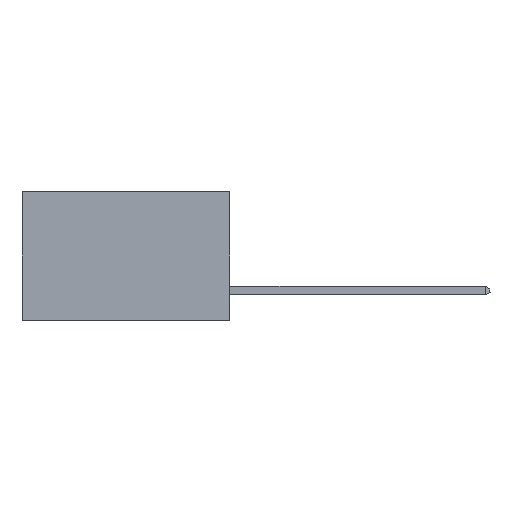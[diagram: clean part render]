
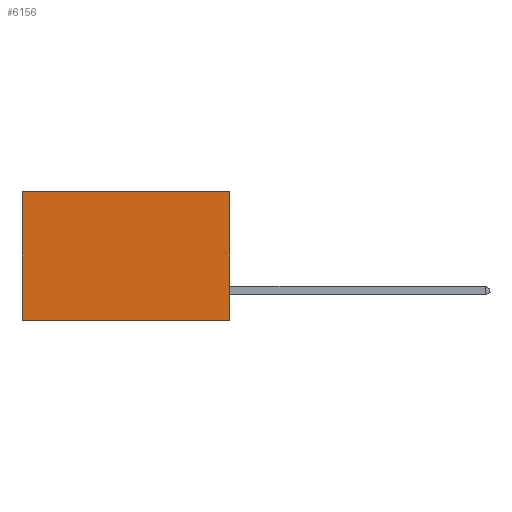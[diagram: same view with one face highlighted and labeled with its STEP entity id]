
A CAD part, left-side view. The second image highlights one B-rep face of the part: STEP entity #6156.
In plain terms, the highlighted planar face has unit normal (-1, 0, 0).
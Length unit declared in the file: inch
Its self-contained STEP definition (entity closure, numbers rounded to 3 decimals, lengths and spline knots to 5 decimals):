
#110 = VERTEX_POINT ( 'NONE', #12939 ) ;
#1541 = EDGE_CURVE ( 'NONE', #110, #9626, #9163, .T. ) ;
#2355 = LINE ( 'NONE', #6905, #5231 ) ;
#3547 = LINE ( 'NONE', #4546, #4515 ) ;
#3570 = CARTESIAN_POINT ( 'NONE',  ( 0.298, 0., -0.37 ) ) ;
#4515 = VECTOR ( 'NONE', #15166, 39.37008 ) ;
#4546 = CARTESIAN_POINT ( 'NONE',  ( 0.298, 0.6, 0. ) ) ;
#4809 = ORIENTED_EDGE ( 'NONE', *, *, #12837, .F. ) ;
#5231 = VECTOR ( 'NONE', #17232, 39.37008 ) ;
#5272 = AXIS2_PLACEMENT_3D ( 'NONE', #15755, #5328, #9803 ) ;
#5328 = DIRECTION ( 'NONE',  ( 1., 0., 0. ) ) ;
#5522 = EDGE_CURVE ( 'NONE', #110, #10022, #7187, .T. ) ;
#6156 = ADVANCED_FACE ( 'NONE', ( #10822 ), #8272, .F. ) ;
#6232 = VERTEX_POINT ( 'NONE', #17664 ) ;
#6905 = CARTESIAN_POINT ( 'NONE',  ( 0.298, 0., -0.37 ) ) ;
#7024 = VECTOR ( 'NONE', #11322, 39.37008 ) ;
#7187 = LINE ( 'NONE', #16234, #12414 ) ;
#8272 = PLANE ( 'NONE',  #5272 ) ;
#9163 = LINE ( 'NONE', #9851, #7024 ) ;
#9521 = CARTESIAN_POINT ( 'NONE',  ( 0.298, 0.6, 0. ) ) ;
#9626 = VERTEX_POINT ( 'NONE', #3570 ) ;
#9778 = ORIENTED_EDGE ( 'NONE', *, *, #1541, .F. ) ;
#9803 = DIRECTION ( 'NONE',  ( 0., 0., -1. ) ) ;
#9851 = CARTESIAN_POINT ( 'NONE',  ( 0.298, 0., 0. ) ) ;
#10022 = VERTEX_POINT ( 'NONE', #9521 ) ;
#10816 = ORIENTED_EDGE ( 'NONE', *, *, #12045, .T. ) ;
#10822 = FACE_OUTER_BOUND ( 'NONE', #11270, .T. ) ;
#11270 = EDGE_LOOP ( 'NONE', ( #10816, #4809, #9778, #15108 ) ) ;
#11322 = DIRECTION ( 'NONE',  ( 0., 0., -1. ) ) ;
#12045 = EDGE_CURVE ( 'NONE', #10022, #6232, #3547, .T. ) ;
#12414 = VECTOR ( 'NONE', #14528, 39.37008 ) ;
#12837 = EDGE_CURVE ( 'NONE', #9626, #6232, #2355, .T. ) ;
#12939 = CARTESIAN_POINT ( 'NONE',  ( 0.298, 0., 0. ) ) ;
#14528 = DIRECTION ( 'NONE',  ( 0., 1., 0. ) ) ;
#15108 = ORIENTED_EDGE ( 'NONE', *, *, #5522, .T. ) ;
#15166 = DIRECTION ( 'NONE',  ( 0., 0., -1. ) ) ;
#15755 = CARTESIAN_POINT ( 'NONE',  ( 0.298, 0., 0. ) ) ;
#16234 = CARTESIAN_POINT ( 'NONE',  ( 0.298, 0., 0. ) ) ;
#17232 = DIRECTION ( 'NONE',  ( 0., 1., 0. ) ) ;
#17664 = CARTESIAN_POINT ( 'NONE',  ( 0.298, 0.6, -0.37 ) ) ;
